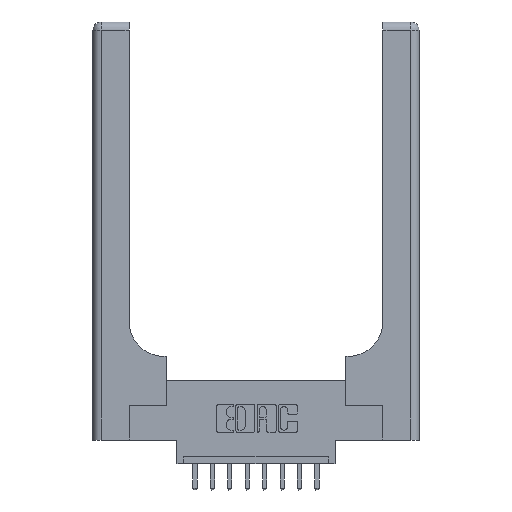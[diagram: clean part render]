
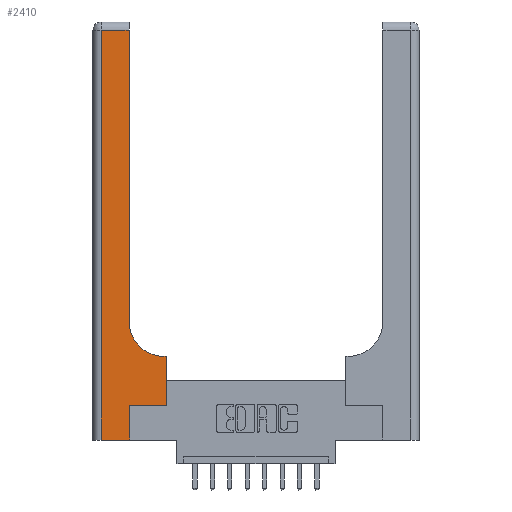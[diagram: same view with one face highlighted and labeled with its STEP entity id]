
A CAD part, top view. The second image highlights one B-rep face of the part: STEP entity #2410.
In plain terms, the highlighted planar face has unit normal (0, 0, 1).
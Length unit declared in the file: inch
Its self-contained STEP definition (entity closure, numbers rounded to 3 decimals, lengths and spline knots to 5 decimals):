
#121 = VECTOR ( 'NONE', #2237, 39.37008 ) ;
#140 = CARTESIAN_POINT ( 'NONE',  ( 0.265, 0., 0.37 ) ) ;
#236 = EDGE_CURVE ( 'NONE', #8876, #13525, #14207, .T. ) ;
#449 = VERTEX_POINT ( 'NONE', #13834 ) ;
#519 = DIRECTION ( 'NONE',  ( -1., 0., 0. ) ) ;
#591 = VECTOR ( 'NONE', #13818, 39.37008 ) ;
#778 = ORIENTED_EDGE ( 'NONE', *, *, #14326, .T. ) ;
#886 = EDGE_CURVE ( 'NONE', #14201, #3632, #4773, .T. ) ;
#1128 = FACE_OUTER_BOUND ( 'NONE', #6139, .T. ) ;
#1133 = EDGE_CURVE ( 'NONE', #5389, #7991, #10560, .T. ) ;
#1656 = DIRECTION ( 'NONE',  ( 0., 0., -1. ) ) ;
#1768 = ORIENTED_EDGE ( 'NONE', *, *, #886, .T. ) ;
#2094 = ORIENTED_EDGE ( 'NONE', *, *, #1133, .T. ) ;
#2237 = DIRECTION ( 'NONE',  ( 0., -1., 0. ) ) ;
#2410 = ADVANCED_FACE ( 'NONE', ( #1128 ), #10834, .F. ) ;
#2437 = CARTESIAN_POINT ( 'NONE',  ( 0.06, 3., 0.37 ) ) ;
#2934 = DIRECTION ( 'NONE',  ( 0., 1., 0. ) ) ;
#3403 = CARTESIAN_POINT ( 'NONE',  ( 0.26, 0.6, 0.37 ) ) ;
#3437 = AXIS2_PLACEMENT_3D ( 'NONE', #10775, #1656, #519 ) ;
#3520 = CARTESIAN_POINT ( 'NONE',  ( 0.51, 0.6, 0.37 ) ) ;
#3632 = VERTEX_POINT ( 'NONE', #13263 ) ;
#3863 = ORIENTED_EDGE ( 'NONE', *, *, #4918, .T. ) ;
#4073 = CARTESIAN_POINT ( 'NONE',  ( 0.528, 0.25, 0.37 ) ) ;
#4274 = LINE ( 'NONE', #2437, #121 ) ;
#4705 = CARTESIAN_POINT ( 'NONE',  ( 0.06, 0., 0.37 ) ) ;
#4773 = LINE ( 'NONE', #14524, #14742 ) ;
#4918 = EDGE_CURVE ( 'NONE', #449, #8876, #14434, .T. ) ;
#5126 = DIRECTION ( 'NONE',  ( 0., 0., -1. ) ) ;
#5157 = VECTOR ( 'NONE', #6478, 39.37008 ) ;
#5369 = VERTEX_POINT ( 'NONE', #4705 ) ;
#5389 = VERTEX_POINT ( 'NONE', #14035 ) ;
#6139 = EDGE_LOOP ( 'NONE', ( #3863, #6444, #6998, #778, #7693, #1768, #8812, #2094, #9331 ) ) ;
#6444 = ORIENTED_EDGE ( 'NONE', *, *, #236, .T. ) ;
#6478 = DIRECTION ( 'NONE',  ( -1., 0., 0. ) ) ;
#6998 = ORIENTED_EDGE ( 'NONE', *, *, #9194, .T. ) ;
#7693 = ORIENTED_EDGE ( 'NONE', *, *, #10209, .T. ) ;
#7991 = VERTEX_POINT ( 'NONE', #3520 ) ;
#8390 = DIRECTION ( 'NONE',  ( 1., 0., 0. ) ) ;
#8812 = ORIENTED_EDGE ( 'NONE', *, *, #9361, .T. ) ;
#8876 = VERTEX_POINT ( 'NONE', #11874 ) ;
#8966 = LINE ( 'NONE', #10291, #14765 ) ;
#9004 = VECTOR ( 'NONE', #8390, 39.37008 ) ;
#9194 = EDGE_CURVE ( 'NONE', #13525, #5369, #4274, .T. ) ;
#9277 = CARTESIAN_POINT ( 'NONE',  ( 0.265, 0.25, 0.37 ) ) ;
#9331 = ORIENTED_EDGE ( 'NONE', *, *, #9755, .T. ) ;
#9361 = EDGE_CURVE ( 'NONE', #3632, #5389, #9888, .T. ) ;
#9755 = EDGE_CURVE ( 'NONE', #7991, #449, #10409, .T. ) ;
#9888 = LINE ( 'NONE', #4073, #12031 ) ;
#10134 = AXIS2_PLACEMENT_3D ( 'NONE', #12028, #5126, #13223 ) ;
#10209 = EDGE_CURVE ( 'NONE', #10382, #14201, #8966, .T. ) ;
#10291 = CARTESIAN_POINT ( 'NONE',  ( 0.265, 0., 0.37 ) ) ;
#10382 = VERTEX_POINT ( 'NONE', #140 ) ;
#10409 = CIRCLE ( 'NONE', #10134, 0.25 ) ;
#10560 = LINE ( 'NONE', #3403, #591 ) ;
#10775 = CARTESIAN_POINT ( 'NONE',  ( 0., 3., 0.37 ) ) ;
#10834 = PLANE ( 'NONE',  #3437 ) ;
#11045 = CARTESIAN_POINT ( 'NONE',  ( 0., 2.94, 0.37 ) ) ;
#11343 = VECTOR ( 'NONE', #14373, 39.37008 ) ;
#11361 = DIRECTION ( 'NONE',  ( 0., 1., 0. ) ) ;
#11874 = CARTESIAN_POINT ( 'NONE',  ( 0.26, 2.94, 0.37 ) ) ;
#12028 = CARTESIAN_POINT ( 'NONE',  ( 0.51, 0.85, 0.37 ) ) ;
#12031 = VECTOR ( 'NONE', #2934, 39.37008 ) ;
#12630 = LINE ( 'NONE', #13156, #9004 ) ;
#13156 = CARTESIAN_POINT ( 'NONE',  ( 0., 0., 0.37 ) ) ;
#13223 = DIRECTION ( 'NONE',  ( 1., 0., 0. ) ) ;
#13263 = CARTESIAN_POINT ( 'NONE',  ( 0.528, 0.25, 0.37 ) ) ;
#13315 = CARTESIAN_POINT ( 'NONE',  ( 0.26, 3., 0.37 ) ) ;
#13413 = DIRECTION ( 'NONE',  ( 1., 0., 0. ) ) ;
#13525 = VERTEX_POINT ( 'NONE', #13638 ) ;
#13638 = CARTESIAN_POINT ( 'NONE',  ( 0.06, 2.94, 0.37 ) ) ;
#13818 = DIRECTION ( 'NONE',  ( -1., 0., 0. ) ) ;
#13834 = CARTESIAN_POINT ( 'NONE',  ( 0.26, 0.85, 0.37 ) ) ;
#14035 = CARTESIAN_POINT ( 'NONE',  ( 0.528, 0.6, 0.37 ) ) ;
#14201 = VERTEX_POINT ( 'NONE', #9277 ) ;
#14207 = LINE ( 'NONE', #11045, #5157 ) ;
#14326 = EDGE_CURVE ( 'NONE', #5369, #10382, #12630, .T. ) ;
#14373 = DIRECTION ( 'NONE',  ( 0., 1., 0. ) ) ;
#14434 = LINE ( 'NONE', #13315, #11343 ) ;
#14524 = CARTESIAN_POINT ( 'NONE',  ( 0.265, 0.25, 0.37 ) ) ;
#14742 = VECTOR ( 'NONE', #13413, 39.37008 ) ;
#14765 = VECTOR ( 'NONE', #11361, 39.37008 ) ;
